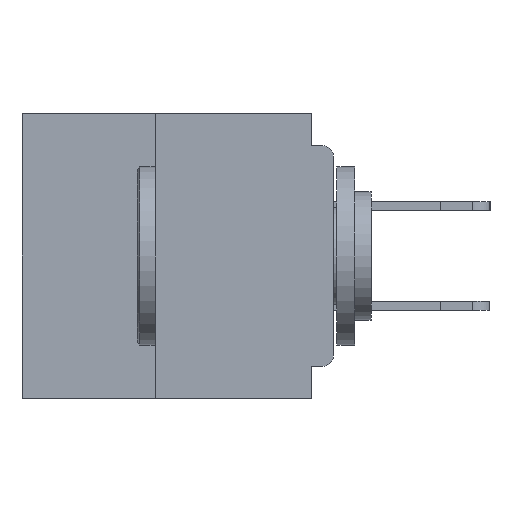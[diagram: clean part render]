
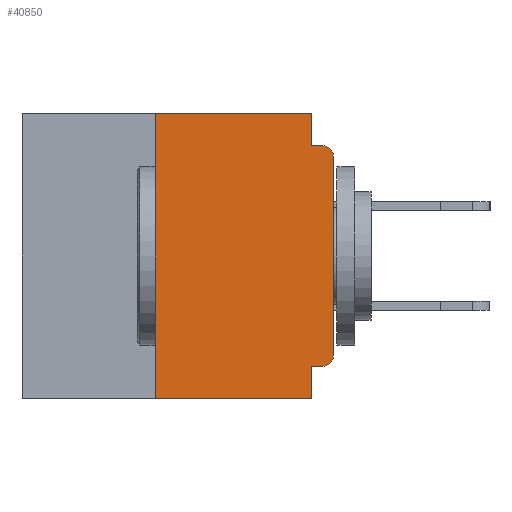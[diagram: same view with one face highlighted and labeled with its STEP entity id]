
A CAD part, left-side view. The second image highlights one B-rep face of the part: STEP entity #40850.
In plain terms, the highlighted planar face has unit normal (-1, 0, 0).
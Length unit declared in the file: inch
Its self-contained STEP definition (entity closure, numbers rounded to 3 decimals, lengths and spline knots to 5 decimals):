
#91 = CARTESIAN_POINT ( 'NONE',  ( 0., 0.25, 0. ) ) ;
#298 = EDGE_LOOP ( 'NONE', ( #4059, #25746, #1701, #9111, #52586, #6024, #38463, #49736, #867, #50742 ) ) ;
#761 = CARTESIAN_POINT ( 'NONE',  ( 0., 0.015, -0.045 ) ) ;
#867 = ORIENTED_EDGE ( 'NONE', *, *, #20192, .F. ) ;
#1701 = ORIENTED_EDGE ( 'NONE', *, *, #15680, .F. ) ;
#1812 = VECTOR ( 'NONE', #52640, 39.37008 ) ;
#2152 = CARTESIAN_POINT ( 'NONE',  ( 0., 0., -0.06 ) ) ;
#2358 = DIRECTION ( 'NONE',  ( 0., 0., -1. ) ) ;
#2895 = DIRECTION ( 'NONE',  ( 0., 0., 1. ) ) ;
#3666 = LINE ( 'NONE', #19569, #46813 ) ;
#3797 = EDGE_CURVE ( 'NONE', #10496, #22007, #38835, .T. ) ;
#4059 = ORIENTED_EDGE ( 'NONE', *, *, #17998, .T. ) ;
#4228 = VECTOR ( 'NONE', #45462, 39.37008 ) ;
#4318 = CARTESIAN_POINT ( 'NONE',  ( 0., 0.031, -0.4 ) ) ;
#5416 = VERTEX_POINT ( 'NONE', #9867 ) ;
#5846 = CIRCLE ( 'NONE', #53276, 0.015 ) ;
#6024 = ORIENTED_EDGE ( 'NONE', *, *, #44830, .F. ) ;
#6588 = CARTESIAN_POINT ( 'NONE',  ( 0., 0.437, 0. ) ) ;
#8011 = CARTESIAN_POINT ( 'NONE',  ( 0., 0.25, -0.4 ) ) ;
#8381 = DIRECTION ( 'NONE',  ( 0., 0., -1. ) ) ;
#9111 = ORIENTED_EDGE ( 'NONE', *, *, #19212, .F. ) ;
#9787 = AXIS2_PLACEMENT_3D ( 'NONE', #10494, #39754, #14705 ) ;
#9867 = CARTESIAN_POINT ( 'NONE',  ( 0., 0.015, -0.355 ) ) ;
#10033 = CARTESIAN_POINT ( 'NONE',  ( 0., 0.031, -0.4 ) ) ;
#10494 = CARTESIAN_POINT ( 'NONE',  ( 0., 0.015, -0.06 ) ) ;
#10496 = VERTEX_POINT ( 'NONE', #91 ) ;
#14406 = CARTESIAN_POINT ( 'NONE',  ( 0., 0.031, 0. ) ) ;
#14705 = DIRECTION ( 'NONE',  ( 0., 0., -1. ) ) ;
#15680 = EDGE_CURVE ( 'NONE', #22846, #41902, #25170, .T. ) ;
#17788 = VECTOR ( 'NONE', #18808, 39.37008 ) ;
#17936 = VECTOR ( 'NONE', #39852, 39.37008 ) ;
#17951 = VECTOR ( 'NONE', #43539, 39.37008 ) ;
#17998 = EDGE_CURVE ( 'NONE', #20353, #24133, #40002, .T. ) ;
#18320 = LINE ( 'NONE', #33314, #29451 ) ;
#18475 = FACE_OUTER_BOUND ( 'NONE', #298, .T. ) ;
#18808 = DIRECTION ( 'NONE',  ( 0., 0., 1. ) ) ;
#19212 = EDGE_CURVE ( 'NONE', #22007, #22846, #18320, .T. ) ;
#19569 = CARTESIAN_POINT ( 'NONE',  ( 0., 0.25, -0.4 ) ) ;
#19609 = LINE ( 'NONE', #23480, #29415 ) ;
#20102 = EDGE_CURVE ( 'NONE', #24133, #41902, #29351, .T. ) ;
#20192 = EDGE_CURVE ( 'NONE', #5416, #26451, #35221, .T. ) ;
#20353 = VERTEX_POINT ( 'NONE', #28802 ) ;
#20493 = CARTESIAN_POINT ( 'NONE',  ( 0., 0., -0.045 ) ) ;
#20876 = DIRECTION ( 'NONE',  ( 1., 0., 0. ) ) ;
#21715 = CARTESIAN_POINT ( 'NONE',  ( 0., 0.031, -0.355 ) ) ;
#22007 = VERTEX_POINT ( 'NONE', #14406 ) ;
#22846 = VERTEX_POINT ( 'NONE', #52993 ) ;
#23480 = CARTESIAN_POINT ( 'NONE',  ( 0., 0.437, -0.4 ) ) ;
#24133 = VERTEX_POINT ( 'NONE', #2152 ) ;
#25170 = LINE ( 'NONE', #20493, #4228 ) ;
#25746 = ORIENTED_EDGE ( 'NONE', *, *, #20102, .T. ) ;
#26451 = VERTEX_POINT ( 'NONE', #21715 ) ;
#27404 = DIRECTION ( 'NONE',  ( -1., 0., 0. ) ) ;
#28802 = CARTESIAN_POINT ( 'NONE',  ( 0., 0., -0.34 ) ) ;
#29287 = CARTESIAN_POINT ( 'NONE',  ( 0., 0.437, 0. ) ) ;
#29351 = CIRCLE ( 'NONE', #9787, 0.015 ) ;
#29415 = VECTOR ( 'NONE', #36110, 39.37008 ) ;
#29451 = VECTOR ( 'NONE', #37484, 39.37008 ) ;
#30450 = AXIS2_PLACEMENT_3D ( 'NONE', #29287, #20876, #8381 ) ;
#32805 = VERTEX_POINT ( 'NONE', #8011 ) ;
#33314 = CARTESIAN_POINT ( 'NONE',  ( 0., 0.031, 0. ) ) ;
#33521 = PLANE ( 'NONE',  #30450 ) ;
#35221 = LINE ( 'NONE', #35946, #1812 ) ;
#35946 = CARTESIAN_POINT ( 'NONE',  ( 0., 0., -0.355 ) ) ;
#36110 = DIRECTION ( 'NONE',  ( 0., -1., 0. ) ) ;
#37484 = DIRECTION ( 'NONE',  ( 0., 0., -1. ) ) ;
#38463 = ORIENTED_EDGE ( 'NONE', *, *, #40049, .T. ) ;
#38531 = VERTEX_POINT ( 'NONE', #4318 ) ;
#38835 = LINE ( 'NONE', #6588, #17936 ) ;
#39754 = DIRECTION ( 'NONE',  ( -1., 0., 0. ) ) ;
#39852 = DIRECTION ( 'NONE',  ( 0., -1., 0. ) ) ;
#40002 = LINE ( 'NONE', #47965, #17788 ) ;
#40049 = EDGE_CURVE ( 'NONE', #32805, #38531, #19609, .T. ) ;
#40850 = ADVANCED_FACE ( 'NONE', ( #18475 ), #33521, .F. ) ;
#41902 = VERTEX_POINT ( 'NONE', #761 ) ;
#42808 = LINE ( 'NONE', #10033, #17951 ) ;
#43539 = DIRECTION ( 'NONE',  ( 0., 0., -1. ) ) ;
#44830 = EDGE_CURVE ( 'NONE', #32805, #10496, #3666, .T. ) ;
#45462 = DIRECTION ( 'NONE',  ( 0., -1., 0. ) ) ;
#46530 = EDGE_CURVE ( 'NONE', #5416, #20353, #5846, .T. ) ;
#46813 = VECTOR ( 'NONE', #2895, 39.37008 ) ;
#47965 = CARTESIAN_POINT ( 'NONE',  ( 0., 0., 0. ) ) ;
#48898 = EDGE_CURVE ( 'NONE', #26451, #38531, #42808, .T. ) ;
#49736 = ORIENTED_EDGE ( 'NONE', *, *, #48898, .F. ) ;
#50742 = ORIENTED_EDGE ( 'NONE', *, *, #46530, .T. ) ;
#52359 = CARTESIAN_POINT ( 'NONE',  ( 0., 0.015, -0.34 ) ) ;
#52586 = ORIENTED_EDGE ( 'NONE', *, *, #3797, .F. ) ;
#52640 = DIRECTION ( 'NONE',  ( 0., 1., 0. ) ) ;
#52993 = CARTESIAN_POINT ( 'NONE',  ( 0., 0.031, -0.045 ) ) ;
#53276 = AXIS2_PLACEMENT_3D ( 'NONE', #52359, #27404, #2358 ) ;
